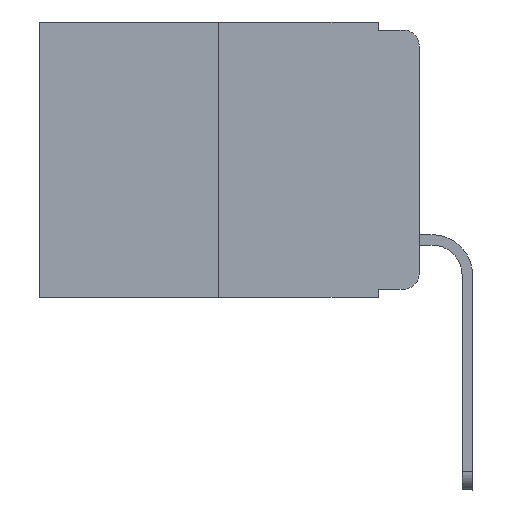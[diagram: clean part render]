
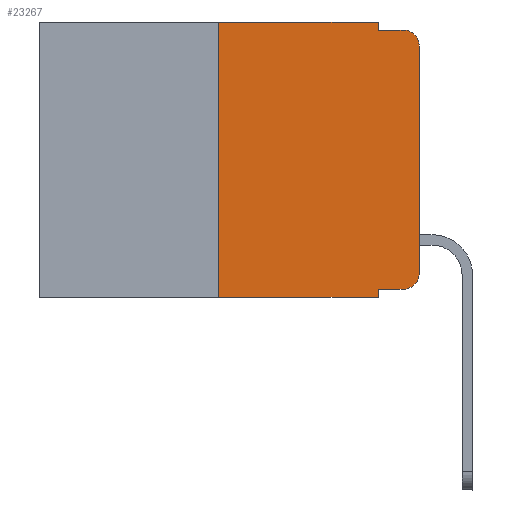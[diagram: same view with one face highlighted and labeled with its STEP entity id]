
A CAD part, left-side view. The second image highlights one B-rep face of the part: STEP entity #23267.
In plain terms, the highlighted planar face has unit normal (-1, 0, 0).
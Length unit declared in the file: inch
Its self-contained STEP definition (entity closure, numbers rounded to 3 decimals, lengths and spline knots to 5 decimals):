
#52 = DIRECTION ( 'NONE',  ( 0., 0., 1. ) ) ;
#71 = CARTESIAN_POINT ( 'NONE',  ( 0., 0.473, 0. ) ) ;
#188 = CIRCLE ( 'NONE', #14964, 0.02 ) ;
#238 = DIRECTION ( 'NONE',  ( 0., -1., 0. ) ) ;
#277 = EDGE_CURVE ( 'NONE', #14019, #3609, #188, .T. ) ;
#498 = VERTEX_POINT ( 'NONE', #1153 ) ;
#1153 = CARTESIAN_POINT ( 'NONE',  ( 0., 0.051, -0.01 ) ) ;
#1522 = EDGE_CURVE ( 'NONE', #4938, #15730, #1910, .T. ) ;
#1789 = VERTEX_POINT ( 'NONE', #6766 ) ;
#1910 = LINE ( 'NONE', #71, #17221 ) ;
#1938 = DIRECTION ( 'NONE',  ( -1., 0., 0. ) ) ;
#2019 = DIRECTION ( 'NONE',  ( 0., -1., 0. ) ) ;
#2379 = CARTESIAN_POINT ( 'NONE',  ( 0., 0.25, 0. ) ) ;
#3078 = ORIENTED_EDGE ( 'NONE', *, *, #21125, .F. ) ;
#3609 = VERTEX_POINT ( 'NONE', #12837 ) ;
#3644 = CARTESIAN_POINT ( 'NONE',  ( 0., 0.02, -0.313 ) ) ;
#4138 = ORIENTED_EDGE ( 'NONE', *, *, #20451, .T. ) ;
#4938 = VERTEX_POINT ( 'NONE', #5423 ) ;
#5423 = CARTESIAN_POINT ( 'NONE',  ( 0., 0.25, 0. ) ) ;
#5615 = CARTESIAN_POINT ( 'NONE',  ( 0., 0.051, -0.01 ) ) ;
#6091 = EDGE_CURVE ( 'NONE', #11909, #9284, #18874, .T. ) ;
#6463 = ORIENTED_EDGE ( 'NONE', *, *, #16913, .F. ) ;
#6475 = CARTESIAN_POINT ( 'NONE',  ( 0., 0.02, -0.333 ) ) ;
#6766 = CARTESIAN_POINT ( 'NONE',  ( 0., 0.25, -0.343 ) ) ;
#7742 = DIRECTION ( 'NONE',  ( 0., 0., 1. ) ) ;
#8441 = AXIS2_PLACEMENT_3D ( 'NONE', #18865, #22892, #17421 ) ;
#8482 = DIRECTION ( 'NONE',  ( -1., 0., 0. ) ) ;
#9215 = CARTESIAN_POINT ( 'NONE',  ( 0., 0., -0.03 ) ) ;
#9284 = VERTEX_POINT ( 'NONE', #12617 ) ;
#9743 = ORIENTED_EDGE ( 'NONE', *, *, #14485, .T. ) ;
#9929 = ORIENTED_EDGE ( 'NONE', *, *, #20079, .T. ) ;
#10246 = CARTESIAN_POINT ( 'NONE',  ( 0., 0.473, -0.343 ) ) ;
#10452 = ORIENTED_EDGE ( 'NONE', *, *, #14950, .F. ) ;
#10751 = VECTOR ( 'NONE', #19285, 39.37008 ) ;
#11357 = ORIENTED_EDGE ( 'NONE', *, *, #277, .T. ) ;
#11468 = FACE_OUTER_BOUND ( 'NONE', #22152, .T. ) ;
#11772 = LINE ( 'NONE', #17359, #10751 ) ;
#11909 = VERTEX_POINT ( 'NONE', #9215 ) ;
#11929 = LINE ( 'NONE', #17615, #18476 ) ;
#12133 = DIRECTION ( 'NONE',  ( 0., 0., -1. ) ) ;
#12508 = CARTESIAN_POINT ( 'NONE',  ( 0., 0.051, -0.333 ) ) ;
#12595 = DIRECTION ( 'NONE',  ( 0., 0., -1. ) ) ;
#12617 = CARTESIAN_POINT ( 'NONE',  ( 0., 0.02, -0.01 ) ) ;
#12837 = CARTESIAN_POINT ( 'NONE',  ( 0., 0., -0.313 ) ) ;
#12873 = LINE ( 'NONE', #16843, #22997 ) ;
#12958 = VERTEX_POINT ( 'NONE', #20151 ) ;
#13776 = DIRECTION ( 'NONE',  ( 0., -1., 0. ) ) ;
#14019 = VERTEX_POINT ( 'NONE', #6475 ) ;
#14123 = LINE ( 'NONE', #10246, #14204 ) ;
#14204 = VECTOR ( 'NONE', #13776, 39.37008 ) ;
#14328 = VERTEX_POINT ( 'NONE', #12508 ) ;
#14485 = EDGE_CURVE ( 'NONE', #3609, #11909, #12873, .T. ) ;
#14768 = CARTESIAN_POINT ( 'NONE',  ( 0., 0.051, 0. ) ) ;
#14867 = LINE ( 'NONE', #5615, #23412 ) ;
#14950 = EDGE_CURVE ( 'NONE', #15730, #498, #19969, .T. ) ;
#14964 = AXIS2_PLACEMENT_3D ( 'NONE', #3644, #1938, #18481 ) ;
#15239 = PLANE ( 'NONE',  #8441 ) ;
#15730 = VERTEX_POINT ( 'NONE', #17617 ) ;
#16843 = CARTESIAN_POINT ( 'NONE',  ( 0., 0., 0. ) ) ;
#16913 = EDGE_CURVE ( 'NONE', #498, #9284, #14867, .T. ) ;
#17098 = LINE ( 'NONE', #2379, #20025 ) ;
#17221 = VECTOR ( 'NONE', #2019, 39.37008 ) ;
#17359 = CARTESIAN_POINT ( 'NONE',  ( 0., 0.051, 0. ) ) ;
#17421 = DIRECTION ( 'NONE',  ( 0., 0., -1. ) ) ;
#17615 = CARTESIAN_POINT ( 'NONE',  ( 0., 0.051, -0.333 ) ) ;
#17617 = CARTESIAN_POINT ( 'NONE',  ( 0., 0.051, 0. ) ) ;
#18192 = CARTESIAN_POINT ( 'NONE',  ( 0., 0.02, -0.03 ) ) ;
#18476 = VECTOR ( 'NONE', #23677, 39.37008 ) ;
#18481 = DIRECTION ( 'NONE',  ( 0., 0., -1. ) ) ;
#18865 = CARTESIAN_POINT ( 'NONE',  ( 0., 0.473, 0. ) ) ;
#18874 = CIRCLE ( 'NONE', #20435, 0.02 ) ;
#19285 = DIRECTION ( 'NONE',  ( 0., 0., -1. ) ) ;
#19383 = ORIENTED_EDGE ( 'NONE', *, *, #6091, .T. ) ;
#19969 = LINE ( 'NONE', #14768, #23345 ) ;
#20025 = VECTOR ( 'NONE', #7742, 39.37008 ) ;
#20079 = EDGE_CURVE ( 'NONE', #1789, #12958, #14123, .T. ) ;
#20151 = CARTESIAN_POINT ( 'NONE',  ( 0., 0.051, -0.343 ) ) ;
#20435 = AXIS2_PLACEMENT_3D ( 'NONE', #18192, #8482, #12133 ) ;
#20451 = EDGE_CURVE ( 'NONE', #14328, #14019, #11929, .T. ) ;
#20596 = EDGE_CURVE ( 'NONE', #1789, #4938, #17098, .T. ) ;
#20693 = ORIENTED_EDGE ( 'NONE', *, *, #1522, .F. ) ;
#21125 = EDGE_CURVE ( 'NONE', #14328, #12958, #11772, .T. ) ;
#22152 = EDGE_LOOP ( 'NONE', ( #9743, #19383, #6463, #10452, #20693, #23496, #9929, #3078, #4138, #11357 ) ) ;
#22892 = DIRECTION ( 'NONE',  ( 1., 0., 0. ) ) ;
#22997 = VECTOR ( 'NONE', #52, 39.37008 ) ;
#23267 = ADVANCED_FACE ( 'NONE', ( #11468 ), #15239, .F. ) ;
#23345 = VECTOR ( 'NONE', #12595, 39.37008 ) ;
#23412 = VECTOR ( 'NONE', #238, 39.37008 ) ;
#23496 = ORIENTED_EDGE ( 'NONE', *, *, #20596, .F. ) ;
#23677 = DIRECTION ( 'NONE',  ( 0., -1., 0. ) ) ;
